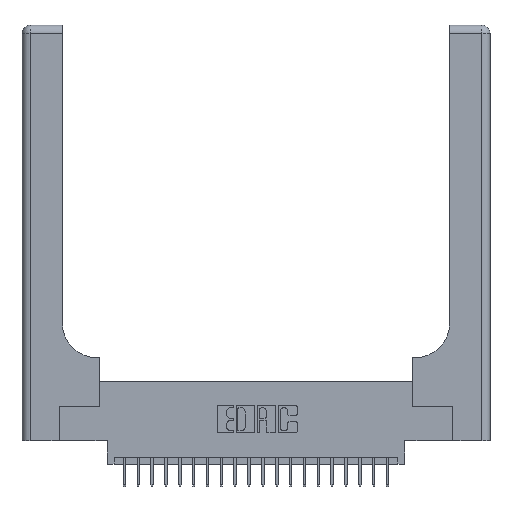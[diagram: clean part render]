
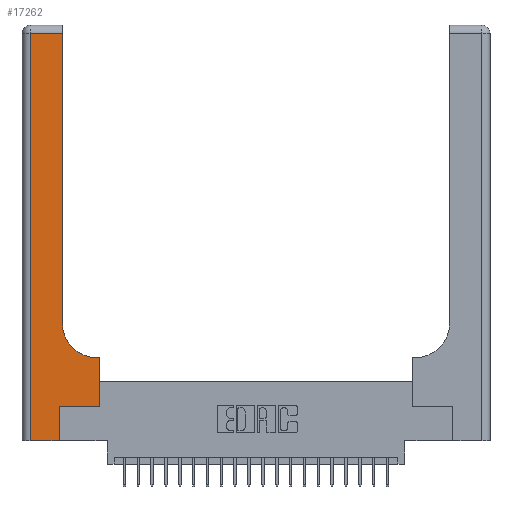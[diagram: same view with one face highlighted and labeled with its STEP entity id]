
A CAD part, top view. The second image highlights one B-rep face of the part: STEP entity #17262.
In plain terms, the highlighted planar face has unit normal (0, 0, 1).
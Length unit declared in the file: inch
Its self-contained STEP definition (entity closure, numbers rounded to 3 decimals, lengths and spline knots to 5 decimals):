
#464 = VERTEX_POINT ( 'NONE', #23603 ) ;
#492 = DIRECTION ( 'NONE',  ( -1., 0., 0. ) ) ;
#818 = VECTOR ( 'NONE', #4317, 39.37008 ) ;
#1041 = DIRECTION ( 'NONE',  ( 0., 1., 0. ) ) ;
#2012 = VECTOR ( 'NONE', #1041, 39.37008 ) ;
#2080 = FACE_OUTER_BOUND ( 'NONE', #20436, .T. ) ;
#2231 = VECTOR ( 'NONE', #22073, 39.37008 ) ;
#2404 = CARTESIAN_POINT ( 'NONE',  ( 0.06, 3., 0.37 ) ) ;
#2528 = ORIENTED_EDGE ( 'NONE', *, *, #3734, .T. ) ;
#2896 = CARTESIAN_POINT ( 'NONE',  ( 0.2915, 0.6, 0.37 ) ) ;
#3274 = VECTOR ( 'NONE', #4783, 39.37008 ) ;
#3543 = LINE ( 'NONE', #16193, #12374 ) ;
#3724 = EDGE_CURVE ( 'NONE', #17435, #12121, #6434, .T. ) ;
#3734 = EDGE_CURVE ( 'NONE', #17586, #17435, #10917, .T. ) ;
#4317 = DIRECTION ( 'NONE',  ( 0., -1., 0. ) ) ;
#4323 = DIRECTION ( 'NONE',  ( 0., 0., -1. ) ) ;
#4783 = DIRECTION ( 'NONE',  ( -1., 0., 0. ) ) ;
#5209 = VECTOR ( 'NONE', #20212, 39.37008 ) ;
#5363 = CARTESIAN_POINT ( 'NONE',  ( 0.06, 2.94, 0.37 ) ) ;
#5480 = EDGE_CURVE ( 'NONE', #12121, #16491, #10286, .T. ) ;
#5545 = DIRECTION ( 'NONE',  ( 0., 0., -1. ) ) ;
#5706 = VERTEX_POINT ( 'NONE', #19173 ) ;
#6434 = LINE ( 'NONE', #2404, #818 ) ;
#6507 = VERTEX_POINT ( 'NONE', #7258 ) ;
#6856 = EDGE_CURVE ( 'NONE', #464, #5706, #12694, .T. ) ;
#6898 = DIRECTION ( 'NONE',  ( 0., 1., 0. ) ) ;
#7258 = CARTESIAN_POINT ( 'NONE',  ( 0.269, 0.25, 0.37 ) ) ;
#7567 = EDGE_CURVE ( 'NONE', #16491, #6507, #3543, .T. ) ;
#7823 = LINE ( 'NONE', #12988, #2231 ) ;
#7923 = CARTESIAN_POINT ( 'NONE',  ( 0.2915, 0.85, 0.37 ) ) ;
#8080 = LINE ( 'NONE', #12786, #17404 ) ;
#10286 = LINE ( 'NONE', #18373, #5209 ) ;
#10800 = CARTESIAN_POINT ( 'NONE',  ( 0.5585, 0.25, 0.37 ) ) ;
#10845 = CARTESIAN_POINT ( 'NONE',  ( 0.06, 0., 0.37 ) ) ;
#10917 = LINE ( 'NONE', #13642, #15190 ) ;
#11320 = CARTESIAN_POINT ( 'NONE',  ( 0.2915, 2.94, 0.37 ) ) ;
#12121 = VERTEX_POINT ( 'NONE', #10845 ) ;
#12374 = VECTOR ( 'NONE', #6898, 39.37008 ) ;
#12694 = LINE ( 'NONE', #2896, #3274 ) ;
#12786 = CARTESIAN_POINT ( 'NONE',  ( 0.269, 0.25, 0.37 ) ) ;
#12832 = ORIENTED_EDGE ( 'NONE', *, *, #5480, .T. ) ;
#12988 = CARTESIAN_POINT ( 'NONE',  ( 0.2915, 3., 0.37 ) ) ;
#13061 = CIRCLE ( 'NONE', #15850, 0.25 ) ;
#13642 = CARTESIAN_POINT ( 'NONE',  ( 0., 2.94, 0.37 ) ) ;
#13651 = CARTESIAN_POINT ( 'NONE',  ( 0., 3., 0.37 ) ) ;
#14170 = CARTESIAN_POINT ( 'NONE',  ( 0.5585, 0.25, 0.37 ) ) ;
#14405 = VERTEX_POINT ( 'NONE', #10800 ) ;
#14482 = EDGE_CURVE ( 'NONE', #6507, #14405, #8080, .T. ) ;
#14726 = ORIENTED_EDGE ( 'NONE', *, *, #19862, .T. ) ;
#15190 = VECTOR ( 'NONE', #492, 39.37008 ) ;
#15491 = PLANE ( 'NONE',  #17670 ) ;
#15850 = AXIS2_PLACEMENT_3D ( 'NONE', #16722, #5545, #18568 ) ;
#16193 = CARTESIAN_POINT ( 'NONE',  ( 0.269, 0., 0.37 ) ) ;
#16284 = ORIENTED_EDGE ( 'NONE', *, *, #7567, .T. ) ;
#16491 = VERTEX_POINT ( 'NONE', #22451 ) ;
#16722 = CARTESIAN_POINT ( 'NONE',  ( 0.5415, 0.85, 0.37 ) ) ;
#17211 = VERTEX_POINT ( 'NONE', #7923 ) ;
#17262 = ADVANCED_FACE ( 'NONE', ( #2080 ), #15491, .F. ) ;
#17366 = DIRECTION ( 'NONE',  ( -1., 0., 0. ) ) ;
#17404 = VECTOR ( 'NONE', #18316, 39.37008 ) ;
#17435 = VERTEX_POINT ( 'NONE', #5363 ) ;
#17586 = VERTEX_POINT ( 'NONE', #11320 ) ;
#17670 = AXIS2_PLACEMENT_3D ( 'NONE', #13651, #4323, #17366 ) ;
#18316 = DIRECTION ( 'NONE',  ( 1., 0., 0. ) ) ;
#18373 = CARTESIAN_POINT ( 'NONE',  ( 0., 0., 0.37 ) ) ;
#18568 = DIRECTION ( 'NONE',  ( 1., 0., 0. ) ) ;
#19173 = CARTESIAN_POINT ( 'NONE',  ( 0.5415, 0.6, 0.37 ) ) ;
#19791 = ORIENTED_EDGE ( 'NONE', *, *, #14482, .T. ) ;
#19862 = EDGE_CURVE ( 'NONE', #14405, #464, #21766, .T. ) ;
#20212 = DIRECTION ( 'NONE',  ( 1., 0., 0. ) ) ;
#20436 = EDGE_LOOP ( 'NONE', ( #23053, #2528, #23945, #12832, #16284, #19791, #14726, #22661, #21277 ) ) ;
#21277 = ORIENTED_EDGE ( 'NONE', *, *, #22428, .T. ) ;
#21318 = EDGE_CURVE ( 'NONE', #17211, #17586, #7823, .T. ) ;
#21766 = LINE ( 'NONE', #14170, #2012 ) ;
#22073 = DIRECTION ( 'NONE',  ( 0., 1., 0. ) ) ;
#22428 = EDGE_CURVE ( 'NONE', #5706, #17211, #13061, .T. ) ;
#22451 = CARTESIAN_POINT ( 'NONE',  ( 0.269, 0., 0.37 ) ) ;
#22661 = ORIENTED_EDGE ( 'NONE', *, *, #6856, .T. ) ;
#23053 = ORIENTED_EDGE ( 'NONE', *, *, #21318, .T. ) ;
#23603 = CARTESIAN_POINT ( 'NONE',  ( 0.5585, 0.6, 0.37 ) ) ;
#23945 = ORIENTED_EDGE ( 'NONE', *, *, #3724, .T. ) ;
